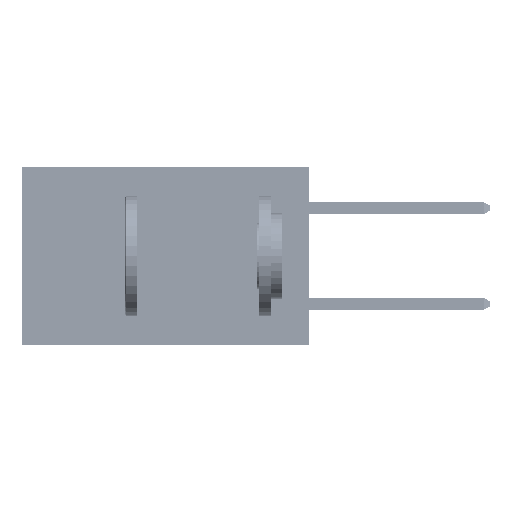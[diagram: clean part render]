
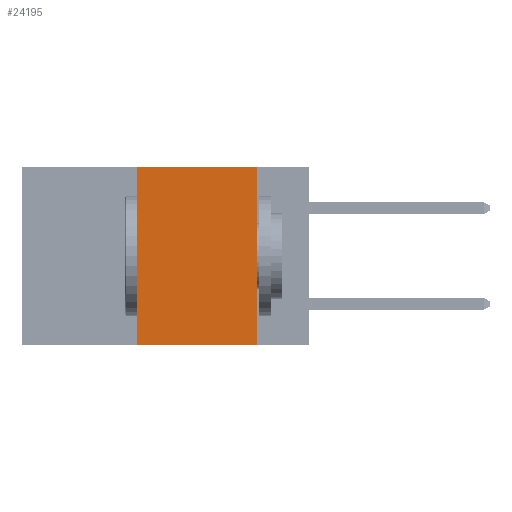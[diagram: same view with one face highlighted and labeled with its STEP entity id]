
A CAD part, left-side view. The second image highlights one B-rep face of the part: STEP entity #24195.
In plain terms, the highlighted planar face has unit normal (-1, 0, 0).
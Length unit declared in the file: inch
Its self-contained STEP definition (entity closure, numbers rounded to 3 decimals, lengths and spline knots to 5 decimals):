
#2647 = VECTOR ( 'NONE', #17496, 39.37008 ) ;
#4176 = DIRECTION ( 'NONE',  ( 0., 0., 1. ) ) ;
#6836 = AXIS2_PLACEMENT_3D ( 'NONE', #41421, #48419, #22367 ) ;
#9185 = LINE ( 'NONE', #36549, #2647 ) ;
#17496 = DIRECTION ( 'NONE',  ( 0., -1., 0. ) ) ;
#19674 = CARTESIAN_POINT ( 'NONE',  ( 0., 0.36, 0. ) ) ;
#19749 = DIRECTION ( 'NONE',  ( 0., -1., 0. ) ) ;
#21549 = ORIENTED_EDGE ( 'NONE', *, *, #25164, .F. ) ;
#22367 = DIRECTION ( 'NONE',  ( 0., 0., -1. ) ) ;
#22406 = LINE ( 'NONE', #36165, #31300 ) ;
#22550 = ORIENTED_EDGE ( 'NONE', *, *, #25972, .T. ) ;
#24195 = ADVANCED_FACE ( 'NONE', ( #28417 ), #48895, .F. ) ;
#24769 = VERTEX_POINT ( 'NONE', #49029 ) ;
#24801 = DIRECTION ( 'NONE',  ( 0., 0., -1. ) ) ;
#25057 = CARTESIAN_POINT ( 'NONE',  ( 0., 0.11, 0. ) ) ;
#25164 = EDGE_CURVE ( 'NONE', #29288, #24769, #22406, .T. ) ;
#25972 = EDGE_CURVE ( 'NONE', #41120, #24769, #45908, .T. ) ;
#26619 = ORIENTED_EDGE ( 'NONE', *, *, #34893, .F. ) ;
#26940 = VECTOR ( 'NONE', #4176, 39.37008 ) ;
#27377 = VECTOR ( 'NONE', #19749, 39.37008 ) ;
#28417 = FACE_OUTER_BOUND ( 'NONE', #30629, .T. ) ;
#29288 = VERTEX_POINT ( 'NONE', #25057 ) ;
#30629 = EDGE_LOOP ( 'NONE', ( #21549, #34584, #26619, #22550 ) ) ;
#31300 = VECTOR ( 'NONE', #24801, 39.37008 ) ;
#31652 = LINE ( 'NONE', #19674, #26940 ) ;
#33139 = EDGE_CURVE ( 'NONE', #43113, #29288, #9185, .T. ) ;
#34584 = ORIENTED_EDGE ( 'NONE', *, *, #33139, .F. ) ;
#34893 = EDGE_CURVE ( 'NONE', #41120, #43113, #31652, .T. ) ;
#35607 = CARTESIAN_POINT ( 'NONE',  ( 0., 0.6, -0.37 ) ) ;
#36165 = CARTESIAN_POINT ( 'NONE',  ( 0., 0.11, 0. ) ) ;
#36549 = CARTESIAN_POINT ( 'NONE',  ( 0., 0.6, 0. ) ) ;
#41120 = VERTEX_POINT ( 'NONE', #45835 ) ;
#41421 = CARTESIAN_POINT ( 'NONE',  ( 0., 0.6, 0. ) ) ;
#43113 = VERTEX_POINT ( 'NONE', #46890 ) ;
#45835 = CARTESIAN_POINT ( 'NONE',  ( 0., 0.36, -0.37 ) ) ;
#45908 = LINE ( 'NONE', #35607, #27377 ) ;
#46890 = CARTESIAN_POINT ( 'NONE',  ( 0., 0.36, 0. ) ) ;
#48419 = DIRECTION ( 'NONE',  ( 1., 0., 0. ) ) ;
#48895 = PLANE ( 'NONE',  #6836 ) ;
#49029 = CARTESIAN_POINT ( 'NONE',  ( 0., 0.11, -0.37 ) ) ;
